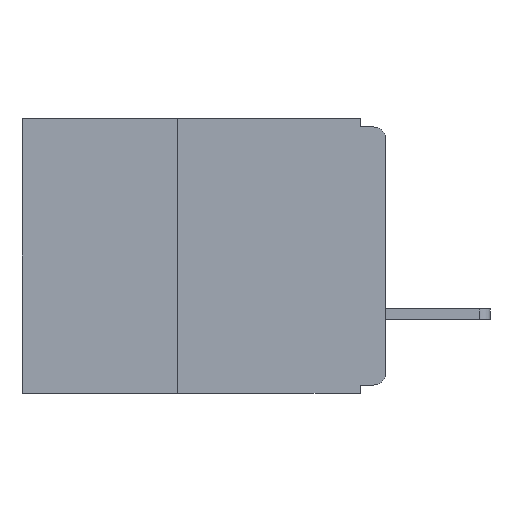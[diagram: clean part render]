
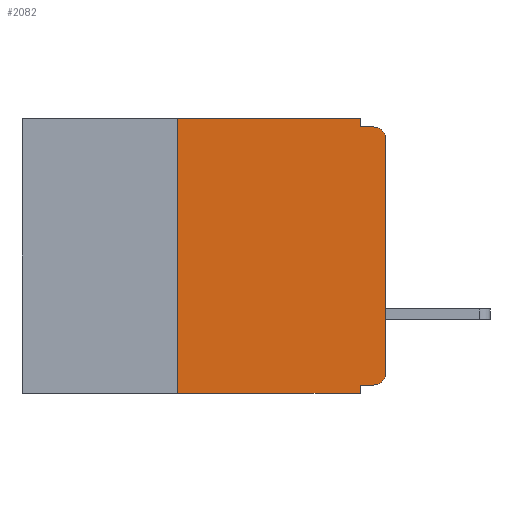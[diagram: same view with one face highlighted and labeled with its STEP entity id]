
A CAD part, left-side view. The second image highlights one B-rep face of the part: STEP entity #2082.
In plain terms, the highlighted planar face has unit normal (-1, 0, 0).
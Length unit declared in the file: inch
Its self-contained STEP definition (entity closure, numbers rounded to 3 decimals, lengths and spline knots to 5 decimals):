
#142 = VECTOR ( 'NONE', #24490, 39.37008 ) ;
#280 = VECTOR ( 'NONE', #4671, 39.37008 ) ;
#414 = CARTESIAN_POINT ( 'NONE',  ( 0., 0.015, -0.32 ) ) ;
#898 = CIRCLE ( 'NONE', #16277, 0.015 ) ;
#1037 = LINE ( 'NONE', #2352, #280 ) ;
#1053 = CARTESIAN_POINT ( 'NONE',  ( 0., 0., -0.305 ) ) ;
#1960 = DIRECTION ( 'NONE',  ( 0., 0., -1. ) ) ;
#2082 = ADVANCED_FACE ( 'NONE', ( #8822 ), #7668, .F. ) ;
#2106 = DIRECTION ( 'NONE',  ( 1., 0., 0. ) ) ;
#2177 = CARTESIAN_POINT ( 'NONE',  ( 0., 0.437, 0. ) ) ;
#2352 = CARTESIAN_POINT ( 'NONE',  ( 0., 0.437, 0. ) ) ;
#2447 = LINE ( 'NONE', #25682, #26432 ) ;
#2507 = VECTOR ( 'NONE', #27405, 39.37008 ) ;
#2662 = CARTESIAN_POINT ( 'NONE',  ( 0., 0.031, 0. ) ) ;
#2697 = AXIS2_PLACEMENT_3D ( 'NONE', #23337, #23325, #23284 ) ;
#2730 = CARTESIAN_POINT ( 'NONE',  ( 0., 0., 0. ) ) ;
#3427 = CARTESIAN_POINT ( 'NONE',  ( 0., 0., -0.025 ) ) ;
#3655 = CARTESIAN_POINT ( 'NONE',  ( 0., 0.25, -0.33 ) ) ;
#3775 = ORIENTED_EDGE ( 'NONE', *, *, #4331, .T. ) ;
#4159 = LINE ( 'NONE', #2730, #22035 ) ;
#4331 = EDGE_CURVE ( 'NONE', #7671, #11803, #25885, .T. ) ;
#4671 = DIRECTION ( 'NONE',  ( 0., -1., 0. ) ) ;
#5533 = LINE ( 'NONE', #2662, #11010 ) ;
#5790 = EDGE_LOOP ( 'NONE', ( #23697, #3775, #7995, #28967, #27949, #24885, #17883, #24453, #25340, #28607 ) ) ;
#5859 = CARTESIAN_POINT ( 'NONE',  ( 0., 0.031, 0. ) ) ;
#6361 = CARTESIAN_POINT ( 'NONE',  ( 0., 0.015, -0.305 ) ) ;
#7426 = VERTEX_POINT ( 'NONE', #8337 ) ;
#7668 = PLANE ( 'NONE',  #19966 ) ;
#7671 = VERTEX_POINT ( 'NONE', #3427 ) ;
#7995 = ORIENTED_EDGE ( 'NONE', *, *, #26137, .F. ) ;
#8078 = VERTEX_POINT ( 'NONE', #414 ) ;
#8337 = CARTESIAN_POINT ( 'NONE',  ( 0., 0.031, -0.01 ) ) ;
#8578 = EDGE_CURVE ( 'NONE', #20032, #7671, #4159, .T. ) ;
#8731 = DIRECTION ( 'NONE',  ( 0., 0., -1. ) ) ;
#8763 = CARTESIAN_POINT ( 'NONE',  ( 0., 0., -0.32 ) ) ;
#8822 = FACE_OUTER_BOUND ( 'NONE', #5790, .T. ) ;
#9937 = CARTESIAN_POINT ( 'NONE',  ( 0., 0.031, -0.33 ) ) ;
#10115 = EDGE_CURVE ( 'NONE', #19716, #19087, #24864, .T. ) ;
#10163 = VECTOR ( 'NONE', #26800, 39.37008 ) ;
#10516 = VERTEX_POINT ( 'NONE', #9937 ) ;
#11010 = VECTOR ( 'NONE', #12026, 39.37008 ) ;
#11197 = CARTESIAN_POINT ( 'NONE',  ( 0., 0.437, -0.33 ) ) ;
#11803 = VERTEX_POINT ( 'NONE', #20468 ) ;
#12026 = DIRECTION ( 'NONE',  ( 0., 0., -1. ) ) ;
#12438 = CARTESIAN_POINT ( 'NONE',  ( 0., 0.031, -0.32 ) ) ;
#12837 = EDGE_CURVE ( 'NONE', #25051, #10516, #22548, .T. ) ;
#14859 = VERTEX_POINT ( 'NONE', #5859 ) ;
#15800 = CARTESIAN_POINT ( 'NONE',  ( 0., 0.25, 0. ) ) ;
#16277 = AXIS2_PLACEMENT_3D ( 'NONE', #6361, #22651, #8731 ) ;
#17883 = ORIENTED_EDGE ( 'NONE', *, *, #25333, .T. ) ;
#18920 = EDGE_CURVE ( 'NONE', #19087, #14859, #1037, .T. ) ;
#18981 = DIRECTION ( 'NONE',  ( 0., 0., 1. ) ) ;
#19087 = VERTEX_POINT ( 'NONE', #15800 ) ;
#19716 = VERTEX_POINT ( 'NONE', #29917 ) ;
#19966 = AXIS2_PLACEMENT_3D ( 'NONE', #2177, #2106, #1960 ) ;
#20032 = VERTEX_POINT ( 'NONE', #1053 ) ;
#20229 = EDGE_CURVE ( 'NONE', #8078, #25051, #29564, .T. ) ;
#20298 = LINE ( 'NONE', #11197, #2507 ) ;
#20416 = DIRECTION ( 'NONE',  ( 0., 1., 0. ) ) ;
#20468 = CARTESIAN_POINT ( 'NONE',  ( 0., 0.015, -0.01 ) ) ;
#22035 = VECTOR ( 'NONE', #18981, 39.37008 ) ;
#22206 = EDGE_CURVE ( 'NONE', #8078, #20032, #898, .T. ) ;
#22548 = LINE ( 'NONE', #24476, #10163 ) ;
#22651 = DIRECTION ( 'NONE',  ( -1., 0., 0. ) ) ;
#23107 = EDGE_CURVE ( 'NONE', #14859, #7426, #5533, .T. ) ;
#23284 = DIRECTION ( 'NONE',  ( 0., 0., -1. ) ) ;
#23325 = DIRECTION ( 'NONE',  ( -1., 0., 0. ) ) ;
#23337 = CARTESIAN_POINT ( 'NONE',  ( 0., 0.015, -0.025 ) ) ;
#23697 = ORIENTED_EDGE ( 'NONE', *, *, #8578, .T. ) ;
#24453 = ORIENTED_EDGE ( 'NONE', *, *, #12837, .F. ) ;
#24476 = CARTESIAN_POINT ( 'NONE',  ( 0., 0.031, -0.33 ) ) ;
#24490 = DIRECTION ( 'NONE',  ( 0., 0., 1. ) ) ;
#24864 = LINE ( 'NONE', #3655, #142 ) ;
#24885 = ORIENTED_EDGE ( 'NONE', *, *, #10115, .F. ) ;
#25051 = VERTEX_POINT ( 'NONE', #12438 ) ;
#25333 = EDGE_CURVE ( 'NONE', #19716, #10516, #20298, .T. ) ;
#25340 = ORIENTED_EDGE ( 'NONE', *, *, #20229, .F. ) ;
#25682 = CARTESIAN_POINT ( 'NONE',  ( 0., 0., -0.01 ) ) ;
#25885 = CIRCLE ( 'NONE', #2697, 0.015 ) ;
#26137 = EDGE_CURVE ( 'NONE', #7426, #11803, #2447, .T. ) ;
#26432 = VECTOR ( 'NONE', #27966, 39.37008 ) ;
#26800 = DIRECTION ( 'NONE',  ( 0., 0., -1. ) ) ;
#27405 = DIRECTION ( 'NONE',  ( 0., -1., 0. ) ) ;
#27949 = ORIENTED_EDGE ( 'NONE', *, *, #18920, .F. ) ;
#27966 = DIRECTION ( 'NONE',  ( 0., -1., 0. ) ) ;
#28607 = ORIENTED_EDGE ( 'NONE', *, *, #22206, .T. ) ;
#28876 = VECTOR ( 'NONE', #20416, 39.37008 ) ;
#28967 = ORIENTED_EDGE ( 'NONE', *, *, #23107, .F. ) ;
#29564 = LINE ( 'NONE', #8763, #28876 ) ;
#29917 = CARTESIAN_POINT ( 'NONE',  ( 0., 0.25, -0.33 ) ) ;
